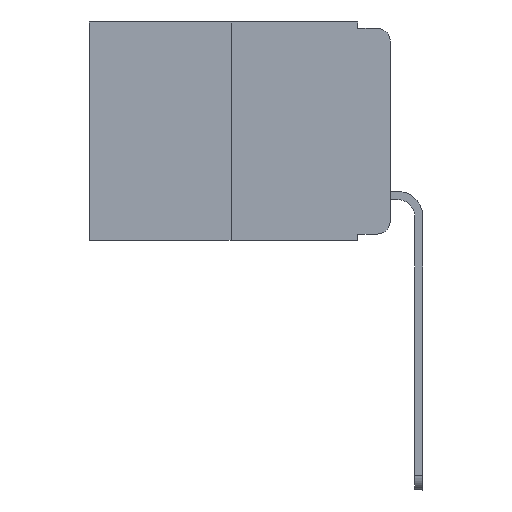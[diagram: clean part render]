
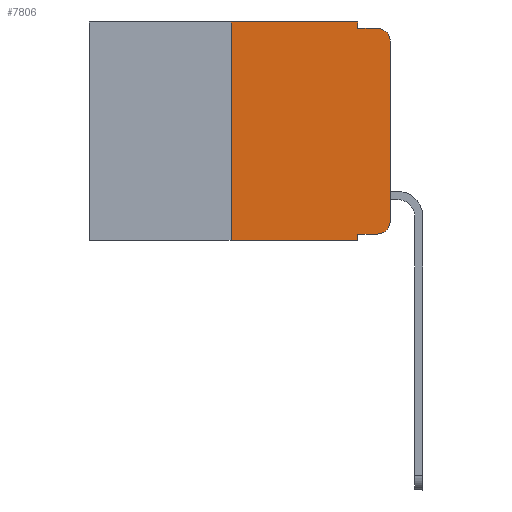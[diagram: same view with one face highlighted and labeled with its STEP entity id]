
A CAD part, left-side view. The second image highlights one B-rep face of the part: STEP entity #7806.
In plain terms, the highlighted planar face has unit normal (-1, 0, 0).
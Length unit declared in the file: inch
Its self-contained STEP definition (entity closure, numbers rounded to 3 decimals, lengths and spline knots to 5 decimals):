
#68 = DIRECTION ( 'NONE',  ( 0., 0., -1. ) ) ;
#539 = AXIS2_PLACEMENT_3D ( 'NONE', #24098, #16911, #68 ) ;
#593 = CARTESIAN_POINT ( 'NONE',  ( 0., 0., -0.313 ) ) ;
#722 = CARTESIAN_POINT ( 'NONE',  ( 0., 0.051, -0.343 ) ) ;
#939 = CARTESIAN_POINT ( 'NONE',  ( 0., 0.473, 0. ) ) ;
#1132 = EDGE_CURVE ( 'NONE', #18173, #22431, #21997, .T. ) ;
#1238 = AXIS2_PLACEMENT_3D ( 'NONE', #8091, #2455, #11617 ) ;
#1714 = LINE ( 'NONE', #5754, #5963 ) ;
#2051 = ORIENTED_EDGE ( 'NONE', *, *, #19865, .T. ) ;
#2455 = DIRECTION ( 'NONE',  ( -1., 0., 0. ) ) ;
#2557 = CARTESIAN_POINT ( 'NONE',  ( 0., 0.051, -0.01 ) ) ;
#3930 = DIRECTION ( 'NONE',  ( 0., 0., 1. ) ) ;
#4024 = ORIENTED_EDGE ( 'NONE', *, *, #6415, .T. ) ;
#4290 = EDGE_CURVE ( 'NONE', #23017, #8865, #22451, .T. ) ;
#4486 = ORIENTED_EDGE ( 'NONE', *, *, #22638, .F. ) ;
#4675 = ORIENTED_EDGE ( 'NONE', *, *, #12744, .T. ) ;
#5244 = AXIS2_PLACEMENT_3D ( 'NONE', #21509, #15929, #12167 ) ;
#5526 = VECTOR ( 'NONE', #20737, 39.37008 ) ;
#5657 = CARTESIAN_POINT ( 'NONE',  ( 0., 0.051, -0.01 ) ) ;
#5754 = CARTESIAN_POINT ( 'NONE',  ( 0., 0., 0. ) ) ;
#5963 = VECTOR ( 'NONE', #3930, 39.37008 ) ;
#6000 = CARTESIAN_POINT ( 'NONE',  ( 0., 0.473, -0.343 ) ) ;
#6306 = ORIENTED_EDGE ( 'NONE', *, *, #4290, .F. ) ;
#6415 = EDGE_CURVE ( 'NONE', #23241, #23148, #1714, .T. ) ;
#7214 = CIRCLE ( 'NONE', #5244, 0.02 ) ;
#7660 = ORIENTED_EDGE ( 'NONE', *, *, #11136, .T. ) ;
#7806 = ADVANCED_FACE ( 'NONE', ( #11327 ), #9506, .F. ) ;
#8091 = CARTESIAN_POINT ( 'NONE',  ( 0., 0.02, -0.313 ) ) ;
#8094 = EDGE_CURVE ( 'NONE', #23148, #12560, #7214, .T. ) ;
#8529 = VERTEX_POINT ( 'NONE', #14526 ) ;
#8665 = CARTESIAN_POINT ( 'NONE',  ( 0., 0.25, -0.343 ) ) ;
#8865 = VERTEX_POINT ( 'NONE', #2557 ) ;
#9428 = CARTESIAN_POINT ( 'NONE',  ( 0., 0.051, 0. ) ) ;
#9506 = PLANE ( 'NONE',  #539 ) ;
#11136 = EDGE_CURVE ( 'NONE', #18173, #23134, #22765, .T. ) ;
#11327 = FACE_OUTER_BOUND ( 'NONE', #24019, .T. ) ;
#11617 = DIRECTION ( 'NONE',  ( 0., 0., -1. ) ) ;
#12007 = ORIENTED_EDGE ( 'NONE', *, *, #1132, .F. ) ;
#12167 = DIRECTION ( 'NONE',  ( 0., 0., -1. ) ) ;
#12207 = CARTESIAN_POINT ( 'NONE',  ( 0., 0., -0.03 ) ) ;
#12560 = VERTEX_POINT ( 'NONE', #15289 ) ;
#12578 = ORIENTED_EDGE ( 'NONE', *, *, #19508, .F. ) ;
#12735 = DIRECTION ( 'NONE',  ( 0., -1., 0. ) ) ;
#12744 = EDGE_CURVE ( 'NONE', #8529, #20211, #18581, .T. ) ;
#12911 = DIRECTION ( 'NONE',  ( 0., 0., 1. ) ) ;
#12977 = CARTESIAN_POINT ( 'NONE',  ( 0., 0.25, 0. ) ) ;
#13064 = CARTESIAN_POINT ( 'NONE',  ( 0., 0.02, -0.333 ) ) ;
#13231 = VECTOR ( 'NONE', #21186, 39.37008 ) ;
#13356 = DIRECTION ( 'NONE',  ( 0., 0., -1. ) ) ;
#14526 = CARTESIAN_POINT ( 'NONE',  ( 0., 0.051, -0.333 ) ) ;
#15289 = CARTESIAN_POINT ( 'NONE',  ( 0., 0.02, -0.01 ) ) ;
#15761 = VECTOR ( 'NONE', #18809, 39.37008 ) ;
#15929 = DIRECTION ( 'NONE',  ( -1., 0., 0. ) ) ;
#16872 = EDGE_CURVE ( 'NONE', #22431, #23017, #17551, .T. ) ;
#16911 = DIRECTION ( 'NONE',  ( 1., 0., 0. ) ) ;
#17326 = VECTOR ( 'NONE', #19280, 39.37008 ) ;
#17399 = VECTOR ( 'NONE', #12735, 39.37008 ) ;
#17542 = ORIENTED_EDGE ( 'NONE', *, *, #8094, .T. ) ;
#17551 = LINE ( 'NONE', #939, #13231 ) ;
#18173 = VERTEX_POINT ( 'NONE', #8665 ) ;
#18390 = CARTESIAN_POINT ( 'NONE',  ( 0., 0.25, 0. ) ) ;
#18581 = LINE ( 'NONE', #23662, #17399 ) ;
#18609 = CARTESIAN_POINT ( 'NONE',  ( 0., 0.051, 0. ) ) ;
#18809 = DIRECTION ( 'NONE',  ( 0., 0., -1. ) ) ;
#19280 = DIRECTION ( 'NONE',  ( 0., -1., 0. ) ) ;
#19508 = EDGE_CURVE ( 'NONE', #8865, #12560, #22307, .T. ) ;
#19865 = EDGE_CURVE ( 'NONE', #20211, #23241, #21837, .T. ) ;
#20211 = VERTEX_POINT ( 'NONE', #13064 ) ;
#20512 = VECTOR ( 'NONE', #12911, 39.37008 ) ;
#20634 = CARTESIAN_POINT ( 'NONE',  ( 0., 0.051, 0. ) ) ;
#20737 = DIRECTION ( 'NONE',  ( 0., -1., 0. ) ) ;
#20864 = LINE ( 'NONE', #20634, #15761 ) ;
#21186 = DIRECTION ( 'NONE',  ( 0., -1., 0. ) ) ;
#21509 = CARTESIAN_POINT ( 'NONE',  ( 0., 0.02, -0.03 ) ) ;
#21837 = CIRCLE ( 'NONE', #1238, 0.02 ) ;
#21997 = LINE ( 'NONE', #18390, #20512 ) ;
#22175 = ORIENTED_EDGE ( 'NONE', *, *, #16872, .F. ) ;
#22307 = LINE ( 'NONE', #5657, #5526 ) ;
#22431 = VERTEX_POINT ( 'NONE', #12977 ) ;
#22451 = LINE ( 'NONE', #18609, #23274 ) ;
#22638 = EDGE_CURVE ( 'NONE', #8529, #23134, #20864, .T. ) ;
#22765 = LINE ( 'NONE', #6000, #17326 ) ;
#23017 = VERTEX_POINT ( 'NONE', #9428 ) ;
#23134 = VERTEX_POINT ( 'NONE', #722 ) ;
#23148 = VERTEX_POINT ( 'NONE', #12207 ) ;
#23241 = VERTEX_POINT ( 'NONE', #593 ) ;
#23274 = VECTOR ( 'NONE', #13356, 39.37008 ) ;
#23662 = CARTESIAN_POINT ( 'NONE',  ( 0., 0.051, -0.333 ) ) ;
#24019 = EDGE_LOOP ( 'NONE', ( #4024, #17542, #12578, #6306, #22175, #12007, #7660, #4486, #4675, #2051 ) ) ;
#24098 = CARTESIAN_POINT ( 'NONE',  ( 0., 0.473, 0. ) ) ;
